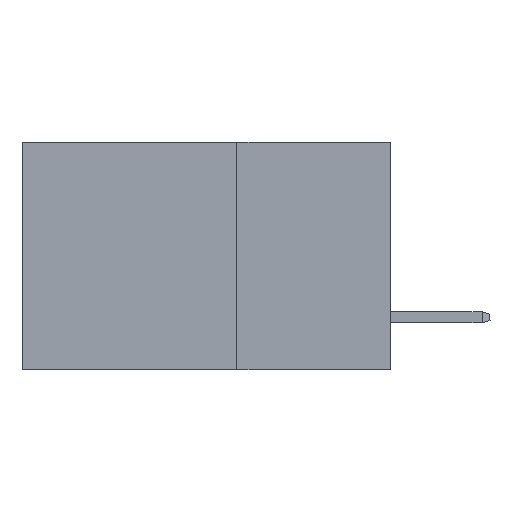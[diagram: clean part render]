
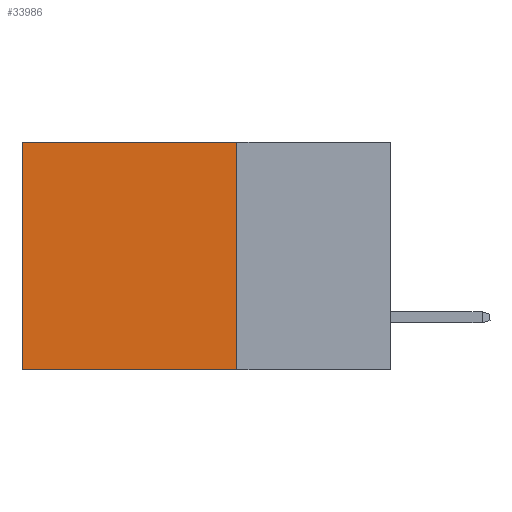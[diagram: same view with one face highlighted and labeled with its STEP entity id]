
A CAD part, left-side view. The second image highlights one B-rep face of the part: STEP entity #33986.
In plain terms, the highlighted planar face has unit normal (-1, 0, 0).
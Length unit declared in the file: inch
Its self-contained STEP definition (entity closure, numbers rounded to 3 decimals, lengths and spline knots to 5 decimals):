
#1011 = CARTESIAN_POINT ( 'NONE',  ( 0.2875, 0.6, 0. ) ) ;
#1743 = EDGE_CURVE ( 'NONE', #6341, #2031, #32608, .T. ) ;
#2031 = VERTEX_POINT ( 'NONE', #36551 ) ;
#2116 = VECTOR ( 'NONE', #3922, 39.37008 ) ;
#3922 = DIRECTION ( 'NONE',  ( 0., 1., 0. ) ) ;
#4336 = ORIENTED_EDGE ( 'NONE', *, *, #8054, .F. ) ;
#4524 = DIRECTION ( 'NONE',  ( 1., 0., 0. ) ) ;
#6341 = VERTEX_POINT ( 'NONE', #36894 ) ;
#7716 = CARTESIAN_POINT ( 'NONE',  ( 0.2875, 0.25, 0. ) ) ;
#8054 = EDGE_CURVE ( 'NONE', #32282, #6341, #19823, .T. ) ;
#10032 = LINE ( 'NONE', #13396, #29195 ) ;
#10217 = CARTESIAN_POINT ( 'NONE',  ( 0.2875, 0.25, 0. ) ) ;
#10384 = VERTEX_POINT ( 'NONE', #1011 ) ;
#11822 = EDGE_LOOP ( 'NONE', ( #13608, #20318, #4336, #18919 ) ) ;
#11935 = AXIS2_PLACEMENT_3D ( 'NONE', #10217, #4524, #33158 ) ;
#12935 = CARTESIAN_POINT ( 'NONE',  ( 0.2875, 0.25, 0. ) ) ;
#13396 = CARTESIAN_POINT ( 'NONE',  ( 0.2875, 0.25, 0. ) ) ;
#13608 = ORIENTED_EDGE ( 'NONE', *, *, #34646, .T. ) ;
#13693 = DIRECTION ( 'NONE',  ( 0., 0., -1. ) ) ;
#15884 = DIRECTION ( 'NONE',  ( 0., 0., -1. ) ) ;
#16647 = CARTESIAN_POINT ( 'NONE',  ( 0.2875, 0.6, 0. ) ) ;
#18315 = CARTESIAN_POINT ( 'NONE',  ( 0.2875, 0.25, -0.37 ) ) ;
#18919 = ORIENTED_EDGE ( 'NONE', *, *, #32826, .T. ) ;
#19823 = LINE ( 'NONE', #12935, #34008 ) ;
#20318 = ORIENTED_EDGE ( 'NONE', *, *, #1743, .F. ) ;
#22098 = DIRECTION ( 'NONE',  ( 0., 1., 0. ) ) ;
#27459 = PLANE ( 'NONE',  #11935 ) ;
#27460 = FACE_OUTER_BOUND ( 'NONE', #11822, .T. ) ;
#28340 = LINE ( 'NONE', #16647, #34129 ) ;
#29195 = VECTOR ( 'NONE', #22098, 39.37008 ) ;
#32282 = VERTEX_POINT ( 'NONE', #7716 ) ;
#32608 = LINE ( 'NONE', #18315, #2116 ) ;
#32826 = EDGE_CURVE ( 'NONE', #32282, #10384, #10032, .T. ) ;
#33158 = DIRECTION ( 'NONE',  ( 0., 0., -1. ) ) ;
#33986 = ADVANCED_FACE ( 'NONE', ( #27460 ), #27459, .F. ) ;
#34008 = VECTOR ( 'NONE', #15884, 39.37008 ) ;
#34129 = VECTOR ( 'NONE', #13693, 39.37008 ) ;
#34646 = EDGE_CURVE ( 'NONE', #10384, #2031, #28340, .T. ) ;
#36551 = CARTESIAN_POINT ( 'NONE',  ( 0.2875, 0.6, -0.37 ) ) ;
#36894 = CARTESIAN_POINT ( 'NONE',  ( 0.2875, 0.25, -0.37 ) ) ;
